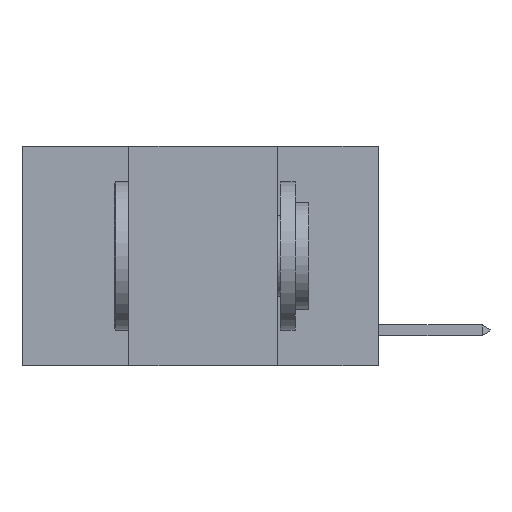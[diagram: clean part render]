
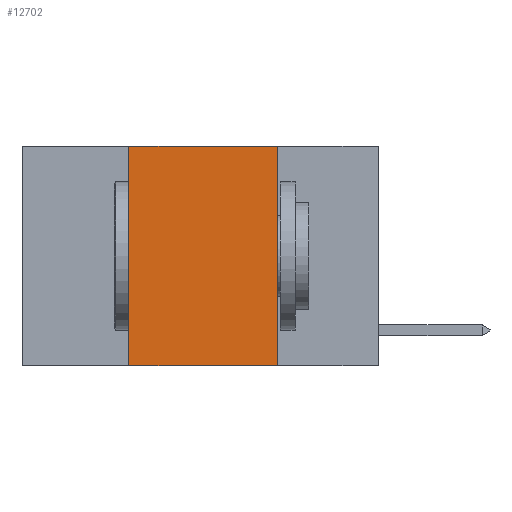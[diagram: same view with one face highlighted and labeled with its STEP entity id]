
A CAD part, left-side view. The second image highlights one B-rep face of the part: STEP entity #12702.
In plain terms, the highlighted planar face has unit normal (-1, 0, 0).
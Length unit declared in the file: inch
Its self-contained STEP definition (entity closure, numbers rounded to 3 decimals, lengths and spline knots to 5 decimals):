
#523 = DIRECTION ( 'NONE',  ( 0., 0., -1. ) ) ;
#1193 = CARTESIAN_POINT ( 'NONE',  ( 0., 0.42, 0. ) ) ;
#1728 = LINE ( 'NONE', #5003, #12276 ) ;
#1984 = LINE ( 'NONE', #4054, #8683 ) ;
#2315 = ORIENTED_EDGE ( 'NONE', *, *, #15134, .F. ) ;
#3259 = EDGE_LOOP ( 'NONE', ( #13153, #11905, #2315, #19792 ) ) ;
#4054 = CARTESIAN_POINT ( 'NONE',  ( 0., 0.17, 0. ) ) ;
#4971 = CARTESIAN_POINT ( 'NONE',  ( 0., 0.17, 0. ) ) ;
#5003 = CARTESIAN_POINT ( 'NONE',  ( 0., 0.6, 0. ) ) ;
#5063 = AXIS2_PLACEMENT_3D ( 'NONE', #8505, #15020, #523 ) ;
#5406 = CARTESIAN_POINT ( 'NONE',  ( 0., 0.17, -0.37 ) ) ;
#7652 = VERTEX_POINT ( 'NONE', #14431 ) ;
#8505 = CARTESIAN_POINT ( 'NONE',  ( 0., 0.6, 0. ) ) ;
#8683 = VECTOR ( 'NONE', #13167, 39.37008 ) ;
#8958 = EDGE_CURVE ( 'NONE', #9682, #11083, #1984, .T. ) ;
#9682 = VERTEX_POINT ( 'NONE', #4971 ) ;
#9913 = DIRECTION ( 'NONE',  ( 0., -1., 0. ) ) ;
#9990 = PLANE ( 'NONE',  #5063 ) ;
#10882 = DIRECTION ( 'NONE',  ( 0., 0., 1. ) ) ;
#11083 = VERTEX_POINT ( 'NONE', #5406 ) ;
#11889 = VECTOR ( 'NONE', #10882, 39.37008 ) ;
#11905 = ORIENTED_EDGE ( 'NONE', *, *, #16520, .F. ) ;
#12276 = VECTOR ( 'NONE', #9913, 39.37008 ) ;
#12693 = CARTESIAN_POINT ( 'NONE',  ( 0., 0.42, -0.37 ) ) ;
#12702 = ADVANCED_FACE ( 'NONE', ( #16305 ), #9990, .F. ) ;
#13153 = ORIENTED_EDGE ( 'NONE', *, *, #8958, .F. ) ;
#13167 = DIRECTION ( 'NONE',  ( 0., 0., -1. ) ) ;
#13772 = LINE ( 'NONE', #20305, #17065 ) ;
#14431 = CARTESIAN_POINT ( 'NONE',  ( 0., 0.42, 0. ) ) ;
#15020 = DIRECTION ( 'NONE',  ( 1., 0., 0. ) ) ;
#15134 = EDGE_CURVE ( 'NONE', #16419, #7652, #17614, .T. ) ;
#16295 = EDGE_CURVE ( 'NONE', #16419, #11083, #13772, .T. ) ;
#16305 = FACE_OUTER_BOUND ( 'NONE', #3259, .T. ) ;
#16419 = VERTEX_POINT ( 'NONE', #12693 ) ;
#16520 = EDGE_CURVE ( 'NONE', #7652, #9682, #1728, .T. ) ;
#17065 = VECTOR ( 'NONE', #18702, 39.37008 ) ;
#17614 = LINE ( 'NONE', #1193, #11889 ) ;
#18702 = DIRECTION ( 'NONE',  ( 0., -1., 0. ) ) ;
#19792 = ORIENTED_EDGE ( 'NONE', *, *, #16295, .T. ) ;
#20305 = CARTESIAN_POINT ( 'NONE',  ( 0., 0.6, -0.37 ) ) ;
